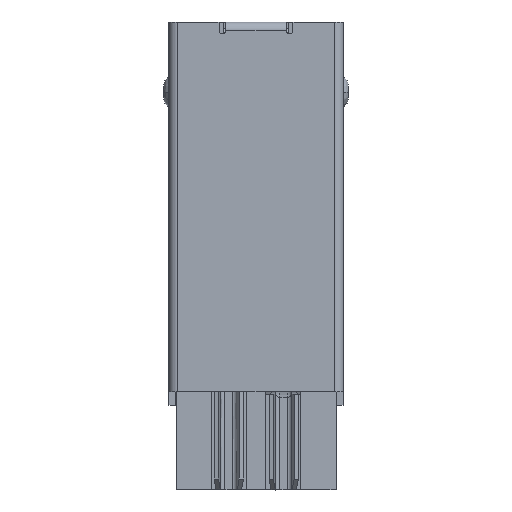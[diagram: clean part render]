
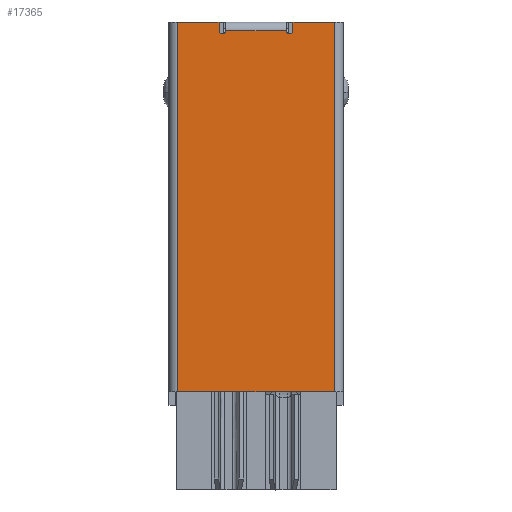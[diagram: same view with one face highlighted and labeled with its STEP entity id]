
A CAD part, front view. The second image highlights one B-rep face of the part: STEP entity #17365.
In plain terms, the highlighted face is planar.
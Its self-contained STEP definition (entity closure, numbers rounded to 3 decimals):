
#46 = AXIS2_PLACEMENT_3D ( 'NONE', #6896, #14342, #12501 ) ;
#132 = CARTESIAN_POINT ( 'NONE',  ( 15.775, 8.618, -0.4 ) ) ;
#251 = DIRECTION ( 'NONE',  ( 0., 1., 0. ) ) ;
#831 = EDGE_CURVE ( 'NONE', #20981, #9103, #4559, .T. ) ;
#928 = CARTESIAN_POINT ( 'NONE',  ( 15.775, 8.618, -8.5 ) ) ;
#1154 = EDGE_CURVE ( 'NONE', #16086, #15961, #20776, .T. ) ;
#1199 = VERTEX_POINT ( 'NONE', #2564 ) ;
#1257 = ORIENTED_EDGE ( 'NONE', *, *, #14786, .T. ) ;
#1554 = ORIENTED_EDGE ( 'NONE', *, *, #18815, .T. ) ;
#1592 = LINE ( 'NONE', #20289, #19277 ) ;
#1638 = PLANE ( 'NONE',  #46 ) ;
#2132 = VERTEX_POINT ( 'NONE', #132 ) ;
#2223 = ORIENTED_EDGE ( 'NONE', *, *, #831, .T. ) ;
#2480 = ORIENTED_EDGE ( 'NONE', *, *, #1154, .T. ) ;
#2564 = CARTESIAN_POINT ( 'NONE',  ( 15.775, 8.768, -0.55 ) ) ;
#2916 = EDGE_CURVE ( 'NONE', #15961, #9380, #1592, .T. ) ;
#3153 = ORIENTED_EDGE ( 'NONE', *, *, #7701, .T. ) ;
#3518 = CARTESIAN_POINT ( 'NONE',  ( 15.775, 12.018, 0. ) ) ;
#3886 = LINE ( 'NONE', #7778, #14937 ) ;
#4013 = CARTESIAN_POINT ( 'NONE',  ( 15.775, 11.718, -0.4 ) ) ;
#4111 = ORIENTED_EDGE ( 'NONE', *, *, #8179, .T. ) ;
#4559 = LINE ( 'NONE', #15438, #17374 ) ;
#4589 = LINE ( 'NONE', #928, #8915 ) ;
#4717 = CIRCLE ( 'NONE', #14865, 0.15 ) ;
#5444 = DIRECTION ( 'NONE',  ( -1., 0., 0. ) ) ;
#5475 = CARTESIAN_POINT ( 'NONE',  ( 15.775, 10.318, 0. ) ) ;
#5525 = CARTESIAN_POINT ( 'NONE',  ( 15.775, 6.718, 0. ) ) ;
#5807 = CARTESIAN_POINT ( 'NONE',  ( 15.775, 6.718, -8.5 ) ) ;
#6065 = VERTEX_POINT ( 'NONE', #4013 ) ;
#6896 = CARTESIAN_POINT ( 'NONE',  ( 15.775, 6.568, -17.34 ) ) ;
#7701 = EDGE_CURVE ( 'NONE', #22613, #16086, #20478, .T. ) ;
#7778 = CARTESIAN_POINT ( 'NONE',  ( 15.775, 10.318, -0.4 ) ) ;
#8179 = EDGE_CURVE ( 'NONE', #20550, #22613, #19826, .T. ) ;
#8915 = VECTOR ( 'NONE', #10071, 1000. ) ;
#8933 = EDGE_LOOP ( 'NONE', ( #1257, #16182, #11309, #21314, #10528, #4111, #3153, #2480, #21794, #1554, #2223 ) ) ;
#9006 = AXIS2_PLACEMENT_3D ( 'NONE', #9300, #24134, #12735 ) ;
#9049 = DIRECTION ( 'NONE',  ( 0., -1., 0. ) ) ;
#9103 = VERTEX_POINT ( 'NONE', #14170 ) ;
#9185 = CARTESIAN_POINT ( 'NONE',  ( 15.775, 11.868, -0.4 ) ) ;
#9300 = CARTESIAN_POINT ( 'NONE',  ( 15.775, 8.768, -0.4 ) ) ;
#9310 = VECTOR ( 'NONE', #9049, 1000. ) ;
#9380 = VERTEX_POINT ( 'NONE', #22862 ) ;
#9526 = CIRCLE ( 'NONE', #17713, 0.15 ) ;
#9563 = VECTOR ( 'NONE', #11417, 1000. ) ;
#10071 = DIRECTION ( 'NONE',  ( 0., 0., 1. ) ) ;
#10511 = CARTESIAN_POINT ( 'NONE',  ( 15.775, 6.718, -17. ) ) ;
#10528 = ORIENTED_EDGE ( 'NONE', *, *, #10718, .T. ) ;
#10718 = EDGE_CURVE ( 'NONE', #2132, #20550, #4589, .T. ) ;
#10909 = CARTESIAN_POINT ( 'NONE',  ( 15.775, 8.618, 0. ) ) ;
#11309 = ORIENTED_EDGE ( 'NONE', *, *, #14723, .T. ) ;
#11417 = DIRECTION ( 'NONE',  ( 0., 0., -1. ) ) ;
#11441 = DIRECTION ( 'NONE',  ( 0., -1., 0. ) ) ;
#11829 = CARTESIAN_POINT ( 'NONE',  ( 15.775, 10.318, -17. ) ) ;
#12501 = DIRECTION ( 'NONE',  ( 0., 1., 0. ) ) ;
#12656 = EDGE_CURVE ( 'NONE', #1199, #2132, #9526, .T. ) ;
#12735 = DIRECTION ( 'NONE',  ( 0., 0., -1. ) ) ;
#12893 = DIRECTION ( 'NONE',  ( 0., 0., -1. ) ) ;
#12926 = DIRECTION ( 'NONE',  ( 0., -1., 0. ) ) ;
#14089 = VECTOR ( 'NONE', #251, 1000. ) ;
#14170 = CARTESIAN_POINT ( 'NONE',  ( 15.775, 12.018, -0.4 ) ) ;
#14342 = DIRECTION ( 'NONE',  ( 1., 0., 0. ) ) ;
#14723 = EDGE_CURVE ( 'NONE', #15338, #1199, #21918, .T. ) ;
#14786 = EDGE_CURVE ( 'NONE', #9103, #6065, #4717, .T. ) ;
#14865 = AXIS2_PLACEMENT_3D ( 'NONE', #9185, #20319, #16755 ) ;
#14937 = VECTOR ( 'NONE', #11441, 1000. ) ;
#15089 = CARTESIAN_POINT ( 'NONE',  ( 15.775, 13.918, -17. ) ) ;
#15338 = VERTEX_POINT ( 'NONE', #19542 ) ;
#15438 = CARTESIAN_POINT ( 'NONE',  ( 15.775, 12.018, -8.5 ) ) ;
#15665 = DIRECTION ( 'NONE',  ( 0., 0., -1. ) ) ;
#15961 = VERTEX_POINT ( 'NONE', #15089 ) ;
#16086 = VERTEX_POINT ( 'NONE', #10511 ) ;
#16172 = FACE_OUTER_BOUND ( 'NONE', #8933, .T. ) ;
#16182 = ORIENTED_EDGE ( 'NONE', *, *, #24103, .T. ) ;
#16755 = DIRECTION ( 'NONE',  ( 0., 0., 1. ) ) ;
#17365 = ADVANCED_FACE ( 'NONE', ( #16172 ), #1638, .T. ) ;
#17374 = VECTOR ( 'NONE', #15665, 1000. ) ;
#17713 = AXIS2_PLACEMENT_3D ( 'NONE', #22451, #5444, #12893 ) ;
#18439 = DIRECTION ( 'NONE',  ( 0., 0., 1. ) ) ;
#18815 = EDGE_CURVE ( 'NONE', #9380, #20981, #23852, .T. ) ;
#19277 = VECTOR ( 'NONE', #18439, 1000. ) ;
#19542 = CARTESIAN_POINT ( 'NONE',  ( 15.775, 8.918, -0.4 ) ) ;
#19826 = LINE ( 'NONE', #23754, #9310 ) ;
#20289 = CARTESIAN_POINT ( 'NONE',  ( 15.775, 13.918, -8.5 ) ) ;
#20319 = DIRECTION ( 'NONE',  ( -1., 0., 0. ) ) ;
#20478 = LINE ( 'NONE', #5807, #9563 ) ;
#20550 = VERTEX_POINT ( 'NONE', #10909 ) ;
#20776 = LINE ( 'NONE', #11829, #14089 ) ;
#20981 = VERTEX_POINT ( 'NONE', #3518 ) ;
#21314 = ORIENTED_EDGE ( 'NONE', *, *, #12656, .T. ) ;
#21794 = ORIENTED_EDGE ( 'NONE', *, *, #2916, .T. ) ;
#21918 = CIRCLE ( 'NONE', #9006, 0.15 ) ;
#22451 = CARTESIAN_POINT ( 'NONE',  ( 15.775, 8.768, -0.4 ) ) ;
#22613 = VERTEX_POINT ( 'NONE', #5525 ) ;
#22708 = VECTOR ( 'NONE', #12926, 1000. ) ;
#22862 = CARTESIAN_POINT ( 'NONE',  ( 15.775, 13.918, 0. ) ) ;
#23754 = CARTESIAN_POINT ( 'NONE',  ( 15.775, 10.318, 0. ) ) ;
#23852 = LINE ( 'NONE', #5475, #22708 ) ;
#24103 = EDGE_CURVE ( 'NONE', #6065, #15338, #3886, .T. ) ;
#24134 = DIRECTION ( 'NONE',  ( -1., 0., 0. ) ) ;
